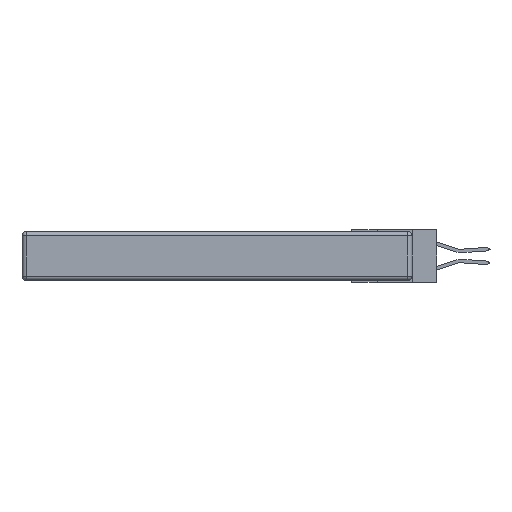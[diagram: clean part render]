
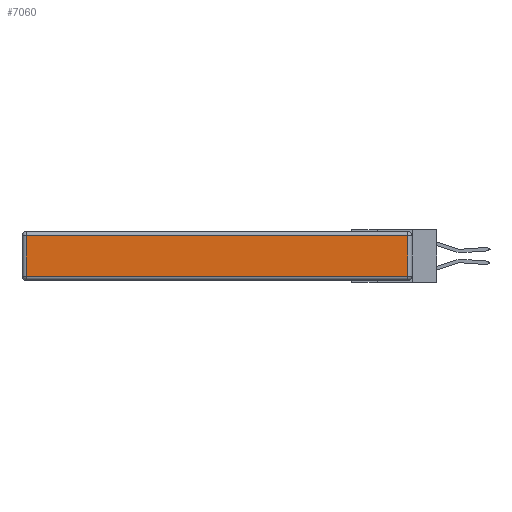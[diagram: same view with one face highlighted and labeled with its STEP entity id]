
A CAD part, left-side view. The second image highlights one B-rep face of the part: STEP entity #7060.
In plain terms, the highlighted planar face has unit normal (-1, 0, 0).
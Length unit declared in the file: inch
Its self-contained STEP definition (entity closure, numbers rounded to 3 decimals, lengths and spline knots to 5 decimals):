
#493 = CARTESIAN_POINT ( 'NONE',  ( 0., 0., -0.313 ) ) ;
#1238 = CARTESIAN_POINT ( 'NONE',  ( 0., 2.72, -0.313 ) ) ;
#1403 = VERTEX_POINT ( 'NONE', #6687 ) ;
#1654 = CARTESIAN_POINT ( 'NONE',  ( 0., 2.72, -0.03 ) ) ;
#1902 = DIRECTION ( 'NONE',  ( 0., -1., 0. ) ) ;
#2227 = VERTEX_POINT ( 'NONE', #1654 ) ;
#3186 = AXIS2_PLACEMENT_3D ( 'NONE', #6736, #9803, #8816 ) ;
#3398 = CARTESIAN_POINT ( 'NONE',  ( 0., 0.03, -0.343 ) ) ;
#3691 = VECTOR ( 'NONE', #10355, 39.37008 ) ;
#4349 = EDGE_LOOP ( 'NONE', ( #13198, #12705, #8229, #4890 ) ) ;
#4847 = EDGE_CURVE ( 'NONE', #12972, #1403, #11145, .T. ) ;
#4882 = CARTESIAN_POINT ( 'NONE',  ( 0., 2.72, -0.343 ) ) ;
#4890 = ORIENTED_EDGE ( 'NONE', *, *, #11176, .T. ) ;
#5123 = VECTOR ( 'NONE', #1902, 39.37008 ) ;
#6687 = CARTESIAN_POINT ( 'NONE',  ( 0., 0.03, -0.313 ) ) ;
#6736 = CARTESIAN_POINT ( 'NONE',  ( 0., 0., -0.343 ) ) ;
#7034 = EDGE_CURVE ( 'NONE', #1403, #8780, #12886, .T. ) ;
#7060 = ADVANCED_FACE ( 'NONE', ( #13209 ), #10819, .T. ) ;
#7128 = CARTESIAN_POINT ( 'NONE',  ( 0., 0.03, -0.03 ) ) ;
#7136 = CARTESIAN_POINT ( 'NONE',  ( 0., 2.75, -0.03 ) ) ;
#7684 = EDGE_CURVE ( 'NONE', #8780, #2227, #10584, .T. ) ;
#7924 = VECTOR ( 'NONE', #10133, 39.37008 ) ;
#8229 = ORIENTED_EDGE ( 'NONE', *, *, #7684, .T. ) ;
#8780 = VERTEX_POINT ( 'NONE', #7128 ) ;
#8816 = DIRECTION ( 'NONE',  ( 0., 0., 1. ) ) ;
#9803 = DIRECTION ( 'NONE',  ( -1., 0., 0. ) ) ;
#10133 = DIRECTION ( 'NONE',  ( 0., 0., -1. ) ) ;
#10355 = DIRECTION ( 'NONE',  ( 0., 1., 0. ) ) ;
#10584 = LINE ( 'NONE', #7136, #3691 ) ;
#10819 = PLANE ( 'NONE',  #3186 ) ;
#11145 = LINE ( 'NONE', #493, #5123 ) ;
#11176 = EDGE_CURVE ( 'NONE', #2227, #12972, #11514, .T. ) ;
#11514 = LINE ( 'NONE', #4882, #7924 ) ;
#11726 = VECTOR ( 'NONE', #12643, 39.37008 ) ;
#12643 = DIRECTION ( 'NONE',  ( 0., 0., 1. ) ) ;
#12705 = ORIENTED_EDGE ( 'NONE', *, *, #7034, .T. ) ;
#12886 = LINE ( 'NONE', #3398, #11726 ) ;
#12972 = VERTEX_POINT ( 'NONE', #1238 ) ;
#13198 = ORIENTED_EDGE ( 'NONE', *, *, #4847, .T. ) ;
#13209 = FACE_OUTER_BOUND ( 'NONE', #4349, .T. ) ;
